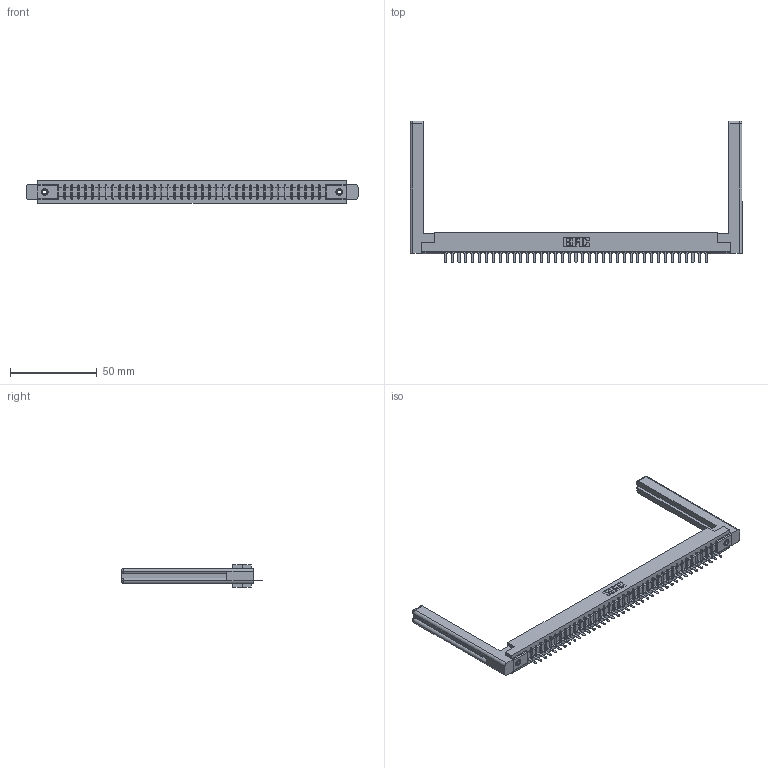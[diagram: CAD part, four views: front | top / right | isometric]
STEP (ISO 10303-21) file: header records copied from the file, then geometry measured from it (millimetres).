
FILE_DESCRIPTION (( 'STEP AP203' ), '1' );
FILE_NAME ('357-039-421-158.STEP', '2020-10-03T04:09:31', ( '' ), ( '' ), 'SwSTEP 2.0', 'SolidWorks 2020', '' );
FILE_SCHEMA (( 'CONFIG_CONTROL_DESIGN' ));
Length unit declared in the file: inch
Products named in the file (5): 307-290-002_521; 357-039-421-158; 307 Part_.156 Dia Mounting Holes; 345-250-001_345-250-001-102; 307-220-058
Assembly tree (44 placements, depth 2):
  357-039-421-158
    307 Part_.156 Dia Mounting Holes
    307-290-002_521  x39
    307-220-058  x2
    345-250-001_345-250-001-102  x2
Bounding box: 191.16 x 81.74 x 12.7 mm (x, y, z)
Volume: 27556.7 mm3; surface area: 30468.6 mm2
Topology: 44 solids, 44 shells, 3186 faces, 9725 edges, 6362 vertices
Faces by surface type: plane 1909, cylinder 1173, sphere 80, torus 12, cone 12
Entity records: 37155 total; most frequent: CARTESIAN_POINT 6275, ORIENTED_EDGE 6204, DIRECTION 6058, EDGE_CURVE 3102, VECTOR 2372, LINE 2372, VERTEX_POINT 2006, AXIS2_PLACEMENT_3D 1843
